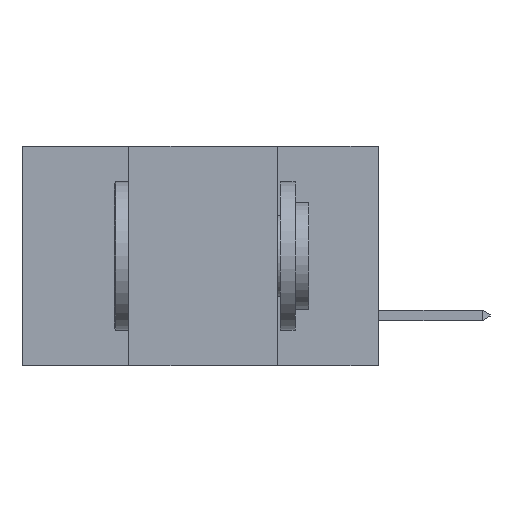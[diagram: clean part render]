
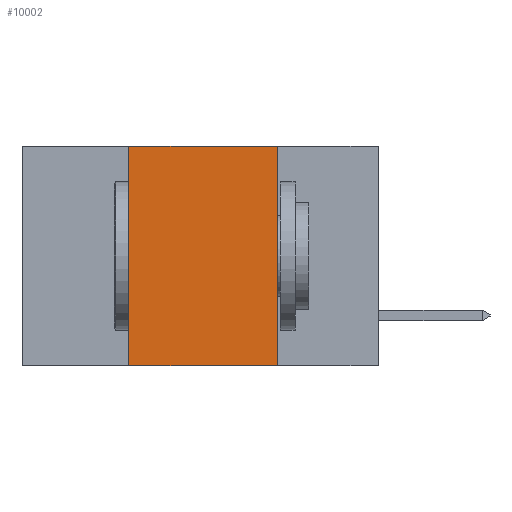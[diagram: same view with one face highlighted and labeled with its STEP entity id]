
A CAD part, left-side view. The second image highlights one B-rep face of the part: STEP entity #10002.
In plain terms, the highlighted planar face has unit normal (-1, 0, 0).
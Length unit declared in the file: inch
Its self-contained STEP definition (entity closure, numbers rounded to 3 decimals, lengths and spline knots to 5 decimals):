
#320 = DIRECTION ( 'NONE',  ( 0., 0., -1. ) ) ;
#1041 = LINE ( 'NONE', #10661, #3914 ) ;
#1782 = DIRECTION ( 'NONE',  ( 1., 0., 0. ) ) ;
#2898 = EDGE_CURVE ( 'NONE', #7169, #7475, #14048, .T. ) ;
#3174 = VERTEX_POINT ( 'NONE', #6604 ) ;
#3703 = ORIENTED_EDGE ( 'NONE', *, *, #12592, .F. ) ;
#3914 = VECTOR ( 'NONE', #10868, 39.37008 ) ;
#4003 = ORIENTED_EDGE ( 'NONE', *, *, #4513, .F. ) ;
#4513 = EDGE_CURVE ( 'NONE', #7475, #3174, #1041, .T. ) ;
#4812 = DIRECTION ( 'NONE',  ( 0., 0., 1. ) ) ;
#5760 = AXIS2_PLACEMENT_3D ( 'NONE', #9061, #1782, #10279 ) ;
#5780 = CARTESIAN_POINT ( 'NONE',  ( 0., 0.42, -0.37 ) ) ;
#6307 = VECTOR ( 'NONE', #7051, 39.37008 ) ;
#6535 = VECTOR ( 'NONE', #320, 39.37008 ) ;
#6604 = CARTESIAN_POINT ( 'NONE',  ( 0., 0.17, 0. ) ) ;
#7051 = DIRECTION ( 'NONE',  ( 0., -1., 0. ) ) ;
#7169 = VERTEX_POINT ( 'NONE', #7344 ) ;
#7344 = CARTESIAN_POINT ( 'NONE',  ( 0., 0.42, -0.37 ) ) ;
#7475 = VERTEX_POINT ( 'NONE', #11536 ) ;
#7544 = CARTESIAN_POINT ( 'NONE',  ( 0., 0.17, -0.37 ) ) ;
#7657 = ORIENTED_EDGE ( 'NONE', *, *, #13635, .T. ) ;
#8352 = VERTEX_POINT ( 'NONE', #13243 ) ;
#8757 = FACE_OUTER_BOUND ( 'NONE', #13018, .T. ) ;
#8971 = ORIENTED_EDGE ( 'NONE', *, *, #2898, .F. ) ;
#9061 = CARTESIAN_POINT ( 'NONE',  ( 0., 0.6, 0. ) ) ;
#9221 = LINE ( 'NONE', #14245, #6307 ) ;
#9447 = LINE ( 'NONE', #7544, #6535 ) ;
#10002 = ADVANCED_FACE ( 'NONE', ( #8757 ), #12625, .F. ) ;
#10279 = DIRECTION ( 'NONE',  ( 0., 0., -1. ) ) ;
#10661 = CARTESIAN_POINT ( 'NONE',  ( 0., 0.6, 0. ) ) ;
#10868 = DIRECTION ( 'NONE',  ( 0., -1., 0. ) ) ;
#10975 = VECTOR ( 'NONE', #4812, 39.37008 ) ;
#11536 = CARTESIAN_POINT ( 'NONE',  ( 0., 0.42, 0. ) ) ;
#12592 = EDGE_CURVE ( 'NONE', #3174, #8352, #9447, .T. ) ;
#12625 = PLANE ( 'NONE',  #5760 ) ;
#13018 = EDGE_LOOP ( 'NONE', ( #3703, #4003, #8971, #7657 ) ) ;
#13243 = CARTESIAN_POINT ( 'NONE',  ( 0., 0.17, -0.37 ) ) ;
#13635 = EDGE_CURVE ( 'NONE', #7169, #8352, #9221, .T. ) ;
#14048 = LINE ( 'NONE', #5780, #10975 ) ;
#14245 = CARTESIAN_POINT ( 'NONE',  ( 0., 0.6, -0.37 ) ) ;
